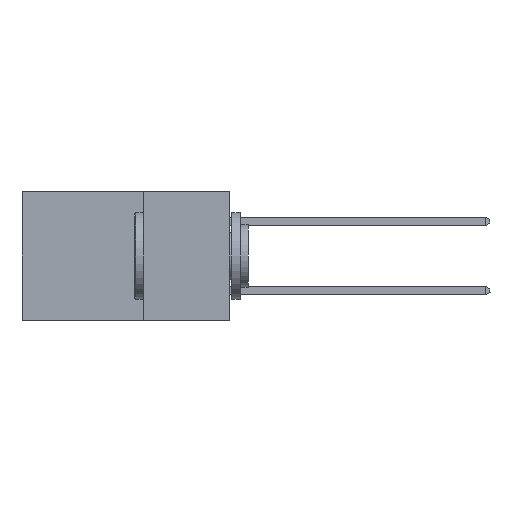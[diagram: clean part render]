
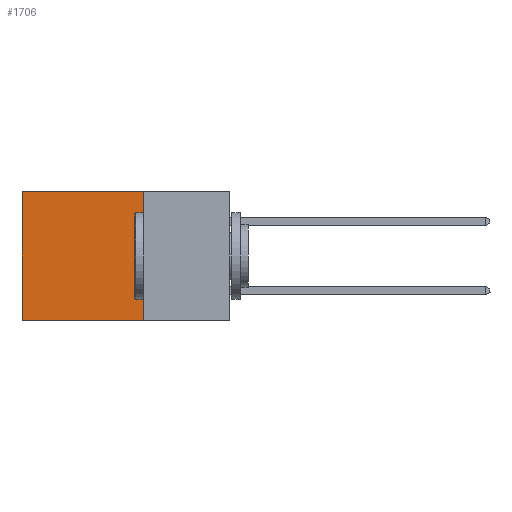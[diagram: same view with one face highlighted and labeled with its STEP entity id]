
A CAD part, left-side view. The second image highlights one B-rep face of the part: STEP entity #1706.
In plain terms, the highlighted planar face has unit normal (-1, 0, 0).
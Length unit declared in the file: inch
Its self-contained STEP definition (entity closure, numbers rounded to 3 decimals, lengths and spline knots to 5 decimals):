
#54 = CARTESIAN_POINT ( 'NONE',  ( 0.298, 0.25, 0. ) ) ;
#98 = VERTEX_POINT ( 'NONE', #5620 ) ;
#1706 = ADVANCED_FACE ( 'NONE', ( #12443 ), #14033, .F. ) ;
#1866 = ORIENTED_EDGE ( 'NONE', *, *, #21093, .F. ) ;
#2766 = EDGE_CURVE ( 'NONE', #98, #14130, #11562, .T. ) ;
#3572 = CARTESIAN_POINT ( 'NONE',  ( 0.298, 0.25, -0.37 ) ) ;
#3662 = DIRECTION ( 'NONE',  ( 0., 0., -1. ) ) ;
#4224 = EDGE_LOOP ( 'NONE', ( #13296, #1866, #19016, #19531 ) ) ;
#5307 = LINE ( 'NONE', #54, #18480 ) ;
#5348 = CARTESIAN_POINT ( 'NONE',  ( 0.298, 0.6, 0. ) ) ;
#5417 = DIRECTION ( 'NONE',  ( 0., 0., -1. ) ) ;
#5620 = CARTESIAN_POINT ( 'NONE',  ( 0.298, 0.25, 0. ) ) ;
#5962 = LINE ( 'NONE', #15957, #16966 ) ;
#6645 = EDGE_CURVE ( 'NONE', #14130, #8354, #5962, .T. ) ;
#7109 = DIRECTION ( 'NONE',  ( 0., 0., -1. ) ) ;
#8354 = VERTEX_POINT ( 'NONE', #15441 ) ;
#8559 = EDGE_CURVE ( 'NONE', #98, #11256, #5307, .T. ) ;
#8917 = CARTESIAN_POINT ( 'NONE',  ( 0.298, 0.25, -0.37 ) ) ;
#10490 = CARTESIAN_POINT ( 'NONE',  ( 0.298, 0.25, 0. ) ) ;
#11256 = VERTEX_POINT ( 'NONE', #8917 ) ;
#11325 = CARTESIAN_POINT ( 'NONE',  ( 0.298, 0.25, 0. ) ) ;
#11562 = LINE ( 'NONE', #11325, #15870 ) ;
#12443 = FACE_OUTER_BOUND ( 'NONE', #4224, .T. ) ;
#12477 = LINE ( 'NONE', #3572, #20801 ) ;
#13296 = ORIENTED_EDGE ( 'NONE', *, *, #6645, .T. ) ;
#13948 = DIRECTION ( 'NONE',  ( 1., 0., 0. ) ) ;
#14033 = PLANE ( 'NONE',  #14376 ) ;
#14130 = VERTEX_POINT ( 'NONE', #5348 ) ;
#14376 = AXIS2_PLACEMENT_3D ( 'NONE', #10490, #13948, #3662 ) ;
#14555 = DIRECTION ( 'NONE',  ( 0., 1., 0. ) ) ;
#15441 = CARTESIAN_POINT ( 'NONE',  ( 0.298, 0.6, -0.37 ) ) ;
#15870 = VECTOR ( 'NONE', #14555, 39.37008 ) ;
#15957 = CARTESIAN_POINT ( 'NONE',  ( 0.298, 0.6, 0. ) ) ;
#16966 = VECTOR ( 'NONE', #7109, 39.37008 ) ;
#18480 = VECTOR ( 'NONE', #5417, 39.37008 ) ;
#19016 = ORIENTED_EDGE ( 'NONE', *, *, #8559, .F. ) ;
#19307 = DIRECTION ( 'NONE',  ( 0., 1., 0. ) ) ;
#19531 = ORIENTED_EDGE ( 'NONE', *, *, #2766, .T. ) ;
#20801 = VECTOR ( 'NONE', #19307, 39.37008 ) ;
#21093 = EDGE_CURVE ( 'NONE', #11256, #8354, #12477, .T. ) ;
